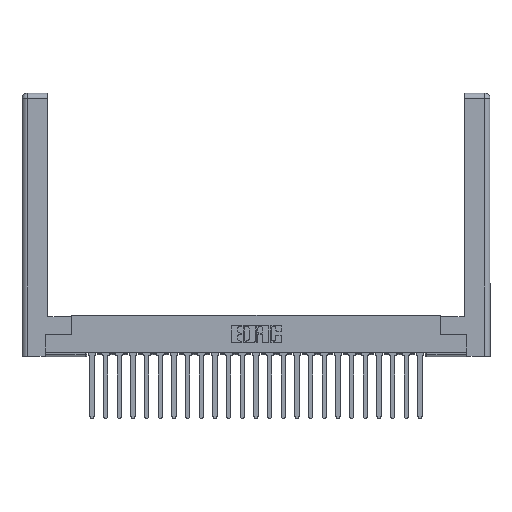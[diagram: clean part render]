
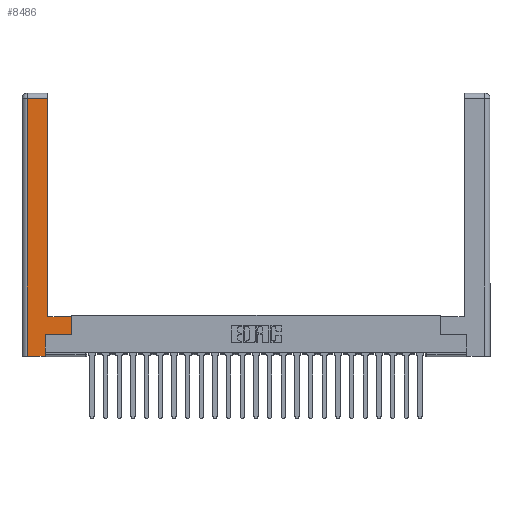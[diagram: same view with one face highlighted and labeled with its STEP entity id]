
A CAD part, top view. The second image highlights one B-rep face of the part: STEP entity #8486.
In plain terms, the highlighted planar face has unit normal (0, 0, 1).
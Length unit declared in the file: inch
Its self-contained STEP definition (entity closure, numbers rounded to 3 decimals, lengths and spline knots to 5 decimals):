
#278 = LINE ( 'NONE', #6589, #20888 ) ;
#315 = VECTOR ( 'NONE', #4964, 39.37008 ) ;
#351 = VERTEX_POINT ( 'NONE', #10002 ) ;
#966 = VERTEX_POINT ( 'NONE', #22734 ) ;
#1490 = CARTESIAN_POINT ( 'NONE',  ( 0.565, 0.245, 0. ) ) ;
#1529 = ORIENTED_EDGE ( 'NONE', *, *, #12142, .T. ) ;
#1589 = LINE ( 'NONE', #5715, #17003 ) ;
#3119 = EDGE_LOOP ( 'NONE', ( #11161, #1529, #3173, #8445, #6719, #17382, #11802, #10546 ) ) ;
#3173 = ORIENTED_EDGE ( 'NONE', *, *, #25224, .T. ) ;
#3906 = EDGE_CURVE ( 'NONE', #15569, #351, #24073, .T. ) ;
#4343 = VECTOR ( 'NONE', #6183, 39.37008 ) ;
#4964 = DIRECTION ( 'NONE',  ( 0., 1., 0. ) ) ;
#4979 = DIRECTION ( 'NONE',  ( -1., 0., 0. ) ) ;
#5102 = CARTESIAN_POINT ( 'NONE',  ( 0.265, 0.245, 0. ) ) ;
#5141 = CARTESIAN_POINT ( 'NONE',  ( 0., 0., 0. ) ) ;
#5640 = VERTEX_POINT ( 'NONE', #7275 ) ;
#5715 = CARTESIAN_POINT ( 'NONE',  ( 0.565, 0.245, 0. ) ) ;
#5880 = VERTEX_POINT ( 'NONE', #1490 ) ;
#5992 = DIRECTION ( 'NONE',  ( 1., 0., 0. ) ) ;
#6183 = DIRECTION ( 'NONE',  ( 0., 1., 0. ) ) ;
#6589 = CARTESIAN_POINT ( 'NONE',  ( 0.265, 0., 0. ) ) ;
#6719 = ORIENTED_EDGE ( 'NONE', *, *, #7038, .T. ) ;
#7038 = EDGE_CURVE ( 'NONE', #966, #24232, #19672, .T. ) ;
#7275 = CARTESIAN_POINT ( 'NONE',  ( 0.0615, 0., 0. ) ) ;
#7281 = AXIS2_PLACEMENT_3D ( 'NONE', #5141, #13464, #9634 ) ;
#7618 = DIRECTION ( 'NONE',  ( 0., 1., 0. ) ) ;
#8445 = ORIENTED_EDGE ( 'NONE', *, *, #18557, .T. ) ;
#8486 = ADVANCED_FACE ( 'NONE', ( #21868 ), #11413, .F. ) ;
#8681 = VECTOR ( 'NONE', #4979, 39.37008 ) ;
#9634 = DIRECTION ( 'NONE',  ( -1., 0., 0. ) ) ;
#9916 = DIRECTION ( 'NONE',  ( -1., 0., 0. ) ) ;
#10002 = CARTESIAN_POINT ( 'NONE',  ( 0.295, 0.45, 0. ) ) ;
#10546 = ORIENTED_EDGE ( 'NONE', *, *, #3906, .T. ) ;
#10608 = DIRECTION ( 'NONE',  ( 0., -1., 0. ) ) ;
#10885 = VECTOR ( 'NONE', #7618, 39.37008 ) ;
#11161 = ORIENTED_EDGE ( 'NONE', *, *, #17673, .T. ) ;
#11389 = CARTESIAN_POINT ( 'NONE',  ( 0.0615, 2.94, 0. ) ) ;
#11413 = PLANE ( 'NONE',  #7281 ) ;
#11789 = VECTOR ( 'NONE', #10608, 39.37008 ) ;
#11802 = ORIENTED_EDGE ( 'NONE', *, *, #12633, .T. ) ;
#12022 = LINE ( 'NONE', #11389, #8681 ) ;
#12142 = EDGE_CURVE ( 'NONE', #22434, #21880, #12022, .T. ) ;
#12174 = VECTOR ( 'NONE', #9916, 39.37008 ) ;
#12633 = EDGE_CURVE ( 'NONE', #5880, #15569, #26017, .T. ) ;
#13464 = DIRECTION ( 'NONE',  ( 0., 0., -1. ) ) ;
#14835 = LINE ( 'NONE', #21054, #11789 ) ;
#15240 = CARTESIAN_POINT ( 'NONE',  ( 0.295, 2.94, 0. ) ) ;
#15569 = VERTEX_POINT ( 'NONE', #19171 ) ;
#15778 = CARTESIAN_POINT ( 'NONE',  ( 0.295, 0.45, 0. ) ) ;
#16122 = CARTESIAN_POINT ( 'NONE',  ( 0.265, 0.245, 0. ) ) ;
#16548 = LINE ( 'NONE', #26882, #4343 ) ;
#17003 = VECTOR ( 'NONE', #5992, 39.37008 ) ;
#17382 = ORIENTED_EDGE ( 'NONE', *, *, #20650, .T. ) ;
#17673 = EDGE_CURVE ( 'NONE', #351, #22434, #16548, .T. ) ;
#18101 = CARTESIAN_POINT ( 'NONE',  ( 0.565, 0.45, 0. ) ) ;
#18557 = EDGE_CURVE ( 'NONE', #5640, #966, #278, .T. ) ;
#19171 = CARTESIAN_POINT ( 'NONE',  ( 0.565, 0.45, 0. ) ) ;
#19672 = LINE ( 'NONE', #5102, #315 ) ;
#20650 = EDGE_CURVE ( 'NONE', #24232, #5880, #1589, .T. ) ;
#20888 = VECTOR ( 'NONE', #21132, 39.37008 ) ;
#21054 = CARTESIAN_POINT ( 'NONE',  ( 0.0615, 0., 0. ) ) ;
#21132 = DIRECTION ( 'NONE',  ( 1., 0., 0. ) ) ;
#21868 = FACE_OUTER_BOUND ( 'NONE', #3119, .T. ) ;
#21880 = VERTEX_POINT ( 'NONE', #24517 ) ;
#22434 = VERTEX_POINT ( 'NONE', #15240 ) ;
#22734 = CARTESIAN_POINT ( 'NONE',  ( 0.265, 0., 0. ) ) ;
#24073 = LINE ( 'NONE', #15778, #12174 ) ;
#24232 = VERTEX_POINT ( 'NONE', #16122 ) ;
#24517 = CARTESIAN_POINT ( 'NONE',  ( 0.0615, 2.94, 0. ) ) ;
#25224 = EDGE_CURVE ( 'NONE', #21880, #5640, #14835, .T. ) ;
#26017 = LINE ( 'NONE', #18101, #10885 ) ;
#26882 = CARTESIAN_POINT ( 'NONE',  ( 0.295, 3., 0. ) ) ;
